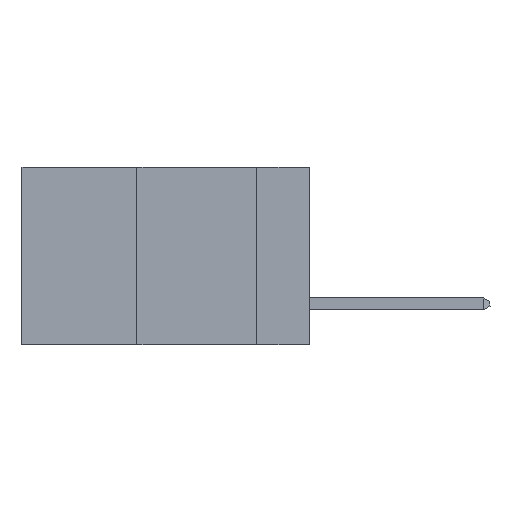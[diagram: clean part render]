
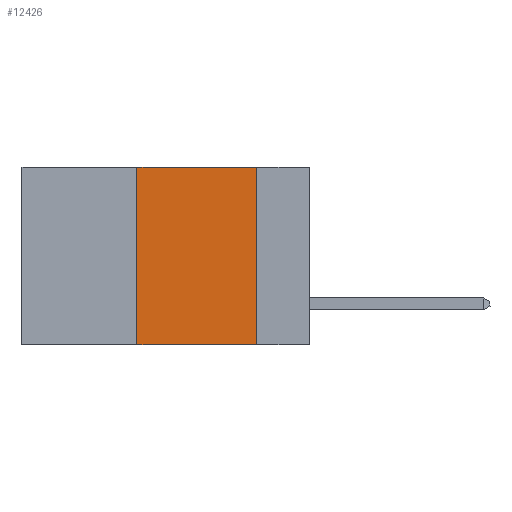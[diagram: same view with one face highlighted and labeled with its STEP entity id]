
A CAD part, left-side view. The second image highlights one B-rep face of the part: STEP entity #12426.
In plain terms, the highlighted planar face has unit normal (-1, 0, 0).
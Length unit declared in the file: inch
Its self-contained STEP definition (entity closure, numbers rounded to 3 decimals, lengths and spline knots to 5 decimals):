
#32 = ORIENTED_EDGE ( 'NONE', *, *, #10219, .F. ) ;
#244 = EDGE_LOOP ( 'NONE', ( #32, #12604, #3211, #739 ) ) ;
#339 = EDGE_CURVE ( 'NONE', #8534, #13562, #3773, .T. ) ;
#660 = CARTESIAN_POINT ( 'NONE',  ( 0., 0.11, 0. ) ) ;
#739 = ORIENTED_EDGE ( 'NONE', *, *, #339, .T. ) ;
#863 = VECTOR ( 'NONE', #4403, 39.37008 ) ;
#1149 = FACE_OUTER_BOUND ( 'NONE', #244, .T. ) ;
#1160 = CARTESIAN_POINT ( 'NONE',  ( 0., 0.6, 0. ) ) ;
#2050 = CARTESIAN_POINT ( 'NONE',  ( 0., 0.36, 0. ) ) ;
#2423 = DIRECTION ( 'NONE',  ( 0., 0., -1. ) ) ;
#2487 = VECTOR ( 'NONE', #3256, 39.37008 ) ;
#2608 = CARTESIAN_POINT ( 'NONE',  ( 0., 0.6, -0.37 ) ) ;
#2782 = DIRECTION ( 'NONE',  ( 0., 0., -1. ) ) ;
#3019 = VECTOR ( 'NONE', #6970, 39.37008 ) ;
#3211 = ORIENTED_EDGE ( 'NONE', *, *, #8095, .F. ) ;
#3256 = DIRECTION ( 'NONE',  ( 0., 0., 1. ) ) ;
#3328 = CARTESIAN_POINT ( 'NONE',  ( 0., 0.11, -0.37 ) ) ;
#3773 = LINE ( 'NONE', #2608, #3019 ) ;
#3926 = EDGE_CURVE ( 'NONE', #5111, #9196, #7245, .T. ) ;
#4403 = DIRECTION ( 'NONE',  ( 0., -1., 0. ) ) ;
#5111 = VERTEX_POINT ( 'NONE', #11429 ) ;
#6444 = CARTESIAN_POINT ( 'NONE',  ( 0., 0.36, -0.37 ) ) ;
#6970 = DIRECTION ( 'NONE',  ( 0., -1., 0. ) ) ;
#7245 = LINE ( 'NONE', #11184, #863 ) ;
#8095 = EDGE_CURVE ( 'NONE', #8534, #5111, #11725, .T. ) ;
#8534 = VERTEX_POINT ( 'NONE', #6444 ) ;
#8600 = CARTESIAN_POINT ( 'NONE',  ( 0., 0.11, 0. ) ) ;
#8996 = VECTOR ( 'NONE', #2782, 39.37008 ) ;
#9196 = VERTEX_POINT ( 'NONE', #660 ) ;
#9424 = DIRECTION ( 'NONE',  ( 1., 0., 0. ) ) ;
#10219 = EDGE_CURVE ( 'NONE', #9196, #13562, #13088, .T. ) ;
#10381 = AXIS2_PLACEMENT_3D ( 'NONE', #1160, #9424, #2423 ) ;
#11184 = CARTESIAN_POINT ( 'NONE',  ( 0., 0.6, 0. ) ) ;
#11429 = CARTESIAN_POINT ( 'NONE',  ( 0., 0.36, 0. ) ) ;
#11725 = LINE ( 'NONE', #2050, #2487 ) ;
#12426 = ADVANCED_FACE ( 'NONE', ( #1149 ), #12803, .F. ) ;
#12604 = ORIENTED_EDGE ( 'NONE', *, *, #3926, .F. ) ;
#12803 = PLANE ( 'NONE',  #10381 ) ;
#13088 = LINE ( 'NONE', #8600, #8996 ) ;
#13562 = VERTEX_POINT ( 'NONE', #3328 ) ;
